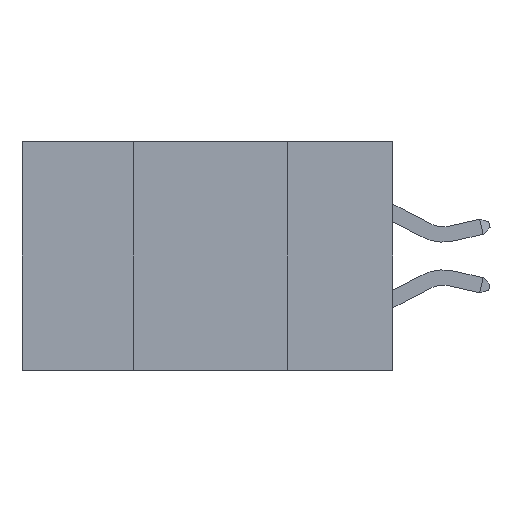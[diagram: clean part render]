
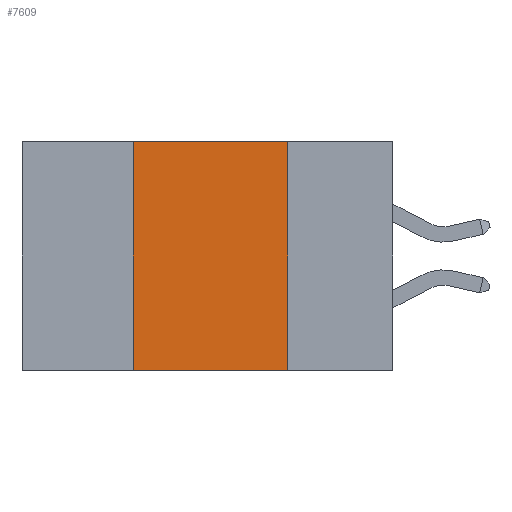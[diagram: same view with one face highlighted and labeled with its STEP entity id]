
A CAD part, left-side view. The second image highlights one B-rep face of the part: STEP entity #7609.
In plain terms, the highlighted planar face has unit normal (-1, 0, 0).
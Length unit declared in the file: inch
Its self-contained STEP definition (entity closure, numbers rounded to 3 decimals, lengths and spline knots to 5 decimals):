
#89 = VECTOR ( 'NONE', #4195, 39.37008 ) ;
#836 = CARTESIAN_POINT ( 'NONE',  ( 0., 0.17, 0. ) ) ;
#1167 = VERTEX_POINT ( 'NONE', #3445 ) ;
#1271 = EDGE_CURVE ( 'NONE', #8436, #8154, #4537, .T. ) ;
#1349 = CARTESIAN_POINT ( 'NONE',  ( 0., 0.6, 0. ) ) ;
#1964 = DIRECTION ( 'NONE',  ( 0., 0., -1. ) ) ;
#2697 = CARTESIAN_POINT ( 'NONE',  ( 0., 0.42, 0. ) ) ;
#3055 = EDGE_CURVE ( 'NONE', #7171, #1167, #6816, .T. ) ;
#3445 = CARTESIAN_POINT ( 'NONE',  ( 0., 0.17, -0.37 ) ) ;
#3559 = ORIENTED_EDGE ( 'NONE', *, *, #1271, .F. ) ;
#3617 = FACE_OUTER_BOUND ( 'NONE', #6930, .T. ) ;
#4050 = CARTESIAN_POINT ( 'NONE',  ( 0., 0.42, 0. ) ) ;
#4163 = LINE ( 'NONE', #7926, #6109 ) ;
#4195 = DIRECTION ( 'NONE',  ( 0., 0., 1. ) ) ;
#4537 = LINE ( 'NONE', #7518, #6909 ) ;
#5257 = CARTESIAN_POINT ( 'NONE',  ( 0., 0.6, -0.37 ) ) ;
#5374 = DIRECTION ( 'NONE',  ( 0., -1., 0. ) ) ;
#5567 = ORIENTED_EDGE ( 'NONE', *, *, #6570, .F. ) ;
#5665 = LINE ( 'NONE', #2697, #89 ) ;
#5887 = DIRECTION ( 'NONE',  ( 1., 0., 0. ) ) ;
#6109 = VECTOR ( 'NONE', #1964, 39.37008 ) ;
#6480 = ORIENTED_EDGE ( 'NONE', *, *, #3055, .T. ) ;
#6570 = EDGE_CURVE ( 'NONE', #7171, #8436, #5665, .T. ) ;
#6816 = LINE ( 'NONE', #5257, #7280 ) ;
#6909 = VECTOR ( 'NONE', #5374, 39.37008 ) ;
#6930 = EDGE_LOOP ( 'NONE', ( #8461, #3559, #5567, #6480 ) ) ;
#7171 = VERTEX_POINT ( 'NONE', #8871 ) ;
#7280 = VECTOR ( 'NONE', #7508, 39.37008 ) ;
#7325 = AXIS2_PLACEMENT_3D ( 'NONE', #1349, #5887, #7446 ) ;
#7446 = DIRECTION ( 'NONE',  ( 0., 0., -1. ) ) ;
#7508 = DIRECTION ( 'NONE',  ( 0., -1., 0. ) ) ;
#7518 = CARTESIAN_POINT ( 'NONE',  ( 0., 0.6, 0. ) ) ;
#7609 = ADVANCED_FACE ( 'NONE', ( #3617 ), #8276, .F. ) ;
#7926 = CARTESIAN_POINT ( 'NONE',  ( 0., 0.17, 0. ) ) ;
#8154 = VERTEX_POINT ( 'NONE', #836 ) ;
#8276 = PLANE ( 'NONE',  #7325 ) ;
#8436 = VERTEX_POINT ( 'NONE', #4050 ) ;
#8461 = ORIENTED_EDGE ( 'NONE', *, *, #9222, .F. ) ;
#8871 = CARTESIAN_POINT ( 'NONE',  ( 0., 0.42, -0.37 ) ) ;
#9222 = EDGE_CURVE ( 'NONE', #8154, #1167, #4163, .T. ) ;
